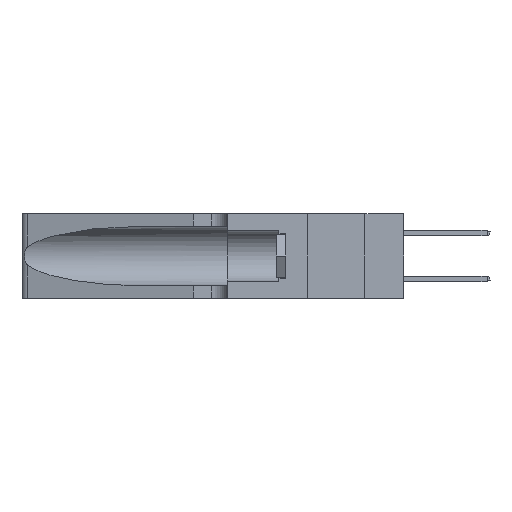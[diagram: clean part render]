
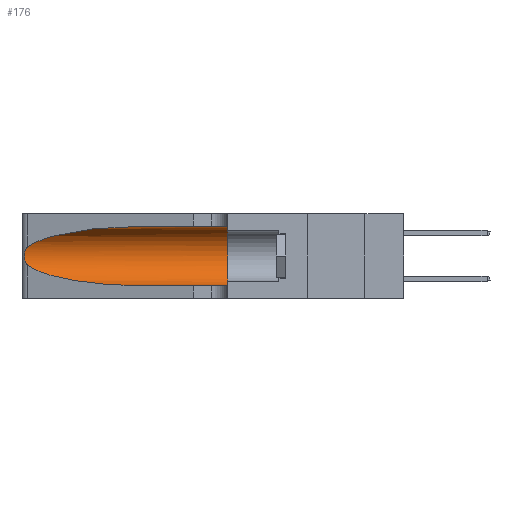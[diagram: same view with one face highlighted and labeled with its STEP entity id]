
A CAD part, left-side view. The second image highlights one B-rep face of the part: STEP entity #176.
In plain terms, the highlighted cylindrical face has radius 3.308 mm (diameter 6.617 mm), a partial arc.
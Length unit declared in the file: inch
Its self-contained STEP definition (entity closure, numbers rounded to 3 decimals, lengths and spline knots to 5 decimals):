
#176 = ADVANCED_FACE ( 'NONE', ( #25316 ), #22550, .F. ) ;
#397 = CARTESIAN_POINT ( 'NONE',  ( 0.1305, 0.72297, 0.05475 ) ) ;
#470 = VECTOR ( 'NONE', #21581, 39.37008 ) ;
#479 = VERTEX_POINT ( 'NONE', #21629 ) ;
#561 = CARTESIAN_POINT ( 'NONE',  ( 0.25487, 1.22718, 0.22369 ) ) ;
#613 = EDGE_CURVE ( 'NONE', #12481, #15060, #21107, .T. ) ;
#1118 = LINE ( 'NONE', #9925, #2843 ) ;
#1406 = CARTESIAN_POINT ( 'NONE',  ( 0.2373, 1.15595, 0.08982 ) ) ;
#1605 = CARTESIAN_POINT ( 'NONE',  ( 0.18966, 0.96281, 0.05475 ) ) ;
#1647 = CARTESIAN_POINT ( 'NONE',  ( 0.1305, 0.72297, 0.31525 ) ) ;
#2843 = VECTOR ( 'NONE', #16409, 39.37008 ) ;
#3394 = EDGE_CURVE ( 'NONE', #479, #15132, #21163, .T. ) ;
#3551 = EDGE_LOOP ( 'NONE', ( #17323, #7726, #6368, #26556, #6209, #14355 ) ) ;
#5114 = CARTESIAN_POINT ( 'NONE',  ( 0.25856, 1.23593, 0.16098 ) ) ;
#5120 = EDGE_CURVE ( 'NONE', #14294, #12481, #15448, .T. ) ;
#6093 = EDGE_CURVE ( 'NONE', #19814, #15060, #1118, .T. ) ;
#6209 = ORIENTED_EDGE ( 'NONE', *, *, #613, .F. ) ;
#6368 = ORIENTED_EDGE ( 'NONE', *, *, #23609, .T. ) ;
#7042 = CARTESIAN_POINT ( 'NONE',  ( 0.25487, 1.22718, 0.14631 ) ) ;
#7726 = ORIENTED_EDGE ( 'NONE', *, *, #3394, .T. ) ;
#8310 = AXIS2_PLACEMENT_3D ( 'NONE', #17937, #22104, #15607 ) ;
#8601 = CARTESIAN_POINT ( 'NONE',  ( 0.1305, 1.61858, 0.31525 ) ) ;
#9733 = CARTESIAN_POINT ( 'NONE',  ( 0.25789, 1.23486, 0.15765 ) ) ;
#9794 = AXIS2_PLACEMENT_3D ( 'NONE', #26720, #10435, #25923 ) ;
#9925 = CARTESIAN_POINT ( 'NONE',  ( 0.1305, 1.61858, 0.05475 ) ) ;
#10336 = CARTESIAN_POINT ( 'NONE',  ( 0.18966, 0.96281, 0.31525 ) ) ;
#10435 = DIRECTION ( 'NONE',  ( 0., -1., 0. ) ) ;
#11664 = CARTESIAN_POINT ( 'NONE',  ( 0.26017, 1.23833, 0.17102 ) ) ;
#11856 = CARTESIAN_POINT ( 'NONE',  ( 0.25487, 1.22718, 0.14631 ) ) ;
#12481 = VERTEX_POINT ( 'NONE', #19550 ) ;
#12597 = CARTESIAN_POINT ( 'NONE',  ( 0.1305, 0.72297, 0.05475 ) ) ;
#14075 = CARTESIAN_POINT ( 'NONE',  ( 0.25639, 1.23186, 0.15144 ) ) ;
#14170 = CARTESIAN_POINT ( 'NONE',  ( 0.25639, 1.23184, 0.21858 ) ) ;
#14294 = VERTEX_POINT ( 'NONE', #1647 ) ;
#14355 = ORIENTED_EDGE ( 'NONE', *, *, #5120, .F. ) ;
#15060 = VERTEX_POINT ( 'NONE', #18101 ) ;
#15132 = VERTEX_POINT ( 'NONE', #7042 ) ;
#15448 = LINE ( 'NONE', #8601, #470 ) ;
#15607 = DIRECTION ( 'NONE',  ( 0., 0., 1. ) ) ;
#16028 =( BOUNDED_CURVE ( )  B_SPLINE_CURVE ( 3, ( #23401, #10336, #16931, #21452 ),
 .UNSPECIFIED., .F., .T. ) 
 B_SPLINE_CURVE_WITH_KNOTS ( ( 4, 4 ),
 ( 1.5708, 2.84003 ),
 .UNSPECIFIED. ) 
 CURVE ( )  GEOMETRIC_REPRESENTATION_ITEM ( )  RATIONAL_B_SPLINE_CURVE ( ( 1., 0.87, 0.87, 1. ) ) 
 REPRESENTATION_ITEM ( '' )  );
#16395 =( BOUNDED_CURVE ( )  B_SPLINE_CURVE ( 3, ( #23736, #1406, #1605, #12597 ),
 .UNSPECIFIED., .F., .F. ) 
 B_SPLINE_CURVE_WITH_KNOTS ( ( 4, 4 ),
 ( 3.44316, 4.71239 ),
 .UNSPECIFIED. ) 
 CURVE ( )  GEOMETRIC_REPRESENTATION_ITEM ( )  RATIONAL_B_SPLINE_CURVE ( ( 1., 0.87, 0.87, 1. ) ) 
 REPRESENTATION_ITEM ( '' )  );
#16409 = DIRECTION ( 'NONE',  ( 0., -1., 0. ) ) ;
#16412 = CARTESIAN_POINT ( 'NONE',  ( 0.25555, 1.22993, 0.14849 ) ) ;
#16931 = CARTESIAN_POINT ( 'NONE',  ( 0.2373, 1.15595, 0.28018 ) ) ;
#17323 = ORIENTED_EDGE ( 'NONE', *, *, #20085, .T. ) ;
#17937 = CARTESIAN_POINT ( 'NONE',  ( 0.1305, 0.35, 0.185 ) ) ;
#18101 = CARTESIAN_POINT ( 'NONE',  ( 0.1305, 0.35, 0.05475 ) ) ;
#18528 = CARTESIAN_POINT ( 'NONE',  ( 0.25854, 1.2359, 0.20912 ) ) ;
#18628 = CARTESIAN_POINT ( 'NONE',  ( 0.26075, 1.23896, 0.178 ) ) ;
#19550 = CARTESIAN_POINT ( 'NONE',  ( 0.1305, 0.35, 0.31525 ) ) ;
#19814 = VERTEX_POINT ( 'NONE', #397 ) ;
#20085 = EDGE_CURVE ( 'NONE', #14294, #479, #16028, .T. ) ;
#21107 = CIRCLE ( 'NONE', #8310, 0.13025 ) ;
#21163 = B_SPLINE_CURVE_WITH_KNOTS ( 'NONE', 3,
 ( #561, #24919, #14170, #22809, #18528, #23097, #27177, #18628, #11664, #5114, #9733, #14075, #16412, #11856 ),
 .UNSPECIFIED., .F., .F.,
 ( 4, 2, 2, 2, 2, 2, 4 ),
 ( 0., 0.00027, 0.00053, 0.00107, 0.0016, 0.00187, 0.00214 ),
 .UNSPECIFIED. ) ;
#21452 = CARTESIAN_POINT ( 'NONE',  ( 0.25487, 1.22718, 0.22369 ) ) ;
#21581 = DIRECTION ( 'NONE',  ( 0., -1., 0. ) ) ;
#21629 = CARTESIAN_POINT ( 'NONE',  ( 0.25487, 1.22718, 0.22369 ) ) ;
#22104 = DIRECTION ( 'NONE',  ( 0., 1., 0. ) ) ;
#22550 = CYLINDRICAL_SURFACE ( 'NONE', #9794, 0.13025 ) ;
#22809 = CARTESIAN_POINT ( 'NONE',  ( 0.25787, 1.23484, 0.2124 ) ) ;
#23097 = CARTESIAN_POINT ( 'NONE',  ( 0.26018, 1.23835, 0.19895 ) ) ;
#23401 = CARTESIAN_POINT ( 'NONE',  ( 0.1305, 0.72297, 0.31525 ) ) ;
#23609 = EDGE_CURVE ( 'NONE', #15132, #19814, #16395, .T. ) ;
#23736 = CARTESIAN_POINT ( 'NONE',  ( 0.25487, 1.22718, 0.14631 ) ) ;
#24919 = CARTESIAN_POINT ( 'NONE',  ( 0.25555, 1.22994, 0.2215 ) ) ;
#25316 = FACE_OUTER_BOUND ( 'NONE', #3551, .T. ) ;
#25923 = DIRECTION ( 'NONE',  ( 0., 0., -1. ) ) ;
#26556 = ORIENTED_EDGE ( 'NONE', *, *, #6093, .T. ) ;
#26720 = CARTESIAN_POINT ( 'NONE',  ( 0.1305, 1.61858, 0.185 ) ) ;
#27177 = CARTESIAN_POINT ( 'NONE',  ( 0.26075, 1.23896, 0.19203 ) ) ;
